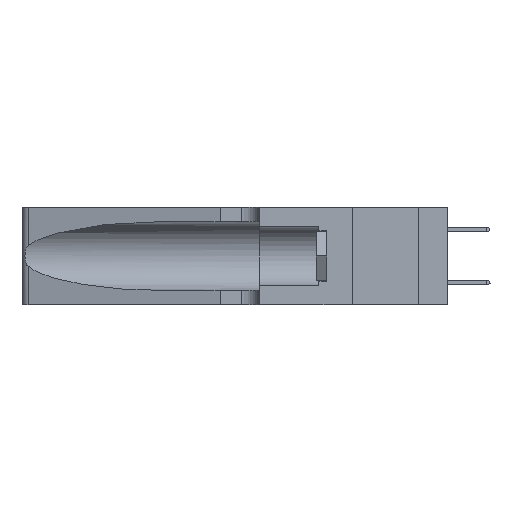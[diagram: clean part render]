
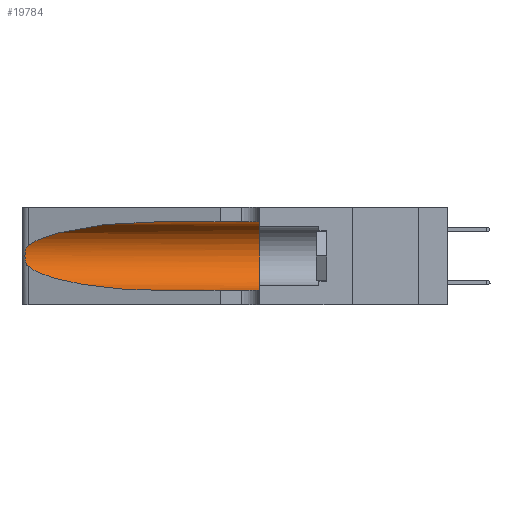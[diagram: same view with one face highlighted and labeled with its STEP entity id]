
A CAD part, left-side view. The second image highlights one B-rep face of the part: STEP entity #19784.
In plain terms, the highlighted cylindrical face has radius 3.308 mm (diameter 6.617 mm), a partial arc.
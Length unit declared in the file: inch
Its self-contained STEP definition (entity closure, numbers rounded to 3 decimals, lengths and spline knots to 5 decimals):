
#1068 = CARTESIAN_POINT ( 'NONE',  ( 0.25856, 1.23593, 0.16098 ) ) ;
#2090 = CARTESIAN_POINT ( 'NONE',  ( 0.1305, 0.35, 0.31525 ) ) ;
#4328 = FACE_OUTER_BOUND ( 'NONE', #12978, .T. ) ;
#4792 = CARTESIAN_POINT ( 'NONE',  ( 0.25487, 1.22718, 0.22369 ) ) ;
#5506 = VERTEX_POINT ( 'NONE', #2090 ) ;
#5895 = EDGE_CURVE ( 'NONE', #29049, #14577, #21340, .T. ) ;
#5913 = CARTESIAN_POINT ( 'NONE',  ( 0.1305, 1.61858, 0.31525 ) ) ;
#6107 = CARTESIAN_POINT ( 'NONE',  ( 0.2373, 1.15595, 0.08982 ) ) ;
#7196 = CARTESIAN_POINT ( 'NONE',  ( 0.25487, 1.22718, 0.22369 ) ) ;
#7689 = CARTESIAN_POINT ( 'NONE',  ( 0.26018, 1.23835, 0.19895 ) ) ;
#8252 = ORIENTED_EDGE ( 'NONE', *, *, #42171, .T. ) ;
#9036 = VECTOR ( 'NONE', #41735, 39.37008 ) ;
#9254 = CARTESIAN_POINT ( 'NONE',  ( 0.2373, 1.15595, 0.28018 ) ) ;
#10290 = CARTESIAN_POINT ( 'NONE',  ( 0.1305, 0.35, 0.185 ) ) ;
#10649 = CARTESIAN_POINT ( 'NONE',  ( 0.25487, 1.22718, 0.22369 ) ) ;
#10930 = CARTESIAN_POINT ( 'NONE',  ( 0.25487, 1.22718, 0.14631 ) ) ;
#11092 = CARTESIAN_POINT ( 'NONE',  ( 0.26075, 1.23896, 0.19203 ) ) ;
#11636 = CARTESIAN_POINT ( 'NONE',  ( 0.1305, 0.72297, 0.05475 ) ) ;
#12978 = EDGE_LOOP ( 'NONE', ( #19654, #16282, #8252, #30655, #33016, #36747 ) ) ;
#13332 = CIRCLE ( 'NONE', #33646, 0.13025 ) ;
#13489 = VERTEX_POINT ( 'NONE', #27936 ) ;
#13955 = CARTESIAN_POINT ( 'NONE',  ( 0.1305, 0.72297, 0.31525 ) ) ;
#13997 = CARTESIAN_POINT ( 'NONE',  ( 0.25639, 1.23186, 0.15144 ) ) ;
#14531 = DIRECTION ( 'NONE',  ( 0., -1., 0. ) ) ;
#14577 = VERTEX_POINT ( 'NONE', #4792 ) ;
#16022 = EDGE_CURVE ( 'NONE', #5506, #13489, #13332, .T. ) ;
#16237 = VECTOR ( 'NONE', #21082, 39.37008 ) ;
#16282 = ORIENTED_EDGE ( 'NONE', *, *, #35152, .T. ) ;
#16532 = DIRECTION ( 'NONE',  ( 0., 1., 0. ) ) ;
#17444 = CARTESIAN_POINT ( 'NONE',  ( 0.25639, 1.23184, 0.21858 ) ) ;
#17752 = CARTESIAN_POINT ( 'NONE',  ( 0.25787, 1.23484, 0.2124 ) ) ;
#18745 = CARTESIAN_POINT ( 'NONE',  ( 0.1305, 0.72297, 0.31525 ) ) ;
#18876 = CARTESIAN_POINT ( 'NONE',  ( 0.25487, 1.22718, 0.14631 ) ) ;
#19654 = ORIENTED_EDGE ( 'NONE', *, *, #5895, .T. ) ;
#19784 = ADVANCED_FACE ( 'NONE', ( #4328 ), #35132, .F. ) ;
#21082 = DIRECTION ( 'NONE',  ( 0., -1., 0. ) ) ;
#21340 =( BOUNDED_CURVE ( )  B_SPLINE_CURVE ( 3, ( #18745, #38522, #9254, #7196 ),
 .UNSPECIFIED., .F., .F. ) 
 B_SPLINE_CURVE_WITH_KNOTS ( ( 4, 4 ),
 ( 1.5708, 2.84003 ),
 .UNSPECIFIED. ) 
 CURVE ( )  GEOMETRIC_REPRESENTATION_ITEM ( )  RATIONAL_B_SPLINE_CURVE ( ( 1., 0.87, 0.87, 1. ) ) 
 REPRESENTATION_ITEM ( '' )  );
#21997 = CARTESIAN_POINT ( 'NONE',  ( 0.1305, 0.72297, 0.05475 ) ) ;
#23235 = DIRECTION ( 'NONE',  ( 0., 0., 1. ) ) ;
#24255 = DIRECTION ( 'NONE',  ( 0., 0., -1. ) ) ;
#24373 = CARTESIAN_POINT ( 'NONE',  ( 0.1305, 1.61858, 0.05475 ) ) ;
#24954 = LINE ( 'NONE', #5913, #9036 ) ;
#25259 = VERTEX_POINT ( 'NONE', #31680 ) ;
#26568 =( BOUNDED_CURVE ( )  B_SPLINE_CURVE ( 3, ( #18876, #6107, #32330, #21997 ),
 .UNSPECIFIED., .F., .F. ) 
 B_SPLINE_CURVE_WITH_KNOTS ( ( 4, 4 ),
 ( 3.44316, 4.71239 ),
 .UNSPECIFIED. ) 
 CURVE ( )  GEOMETRIC_REPRESENTATION_ITEM ( )  RATIONAL_B_SPLINE_CURVE ( ( 1., 0.87, 0.87, 1. ) ) 
 REPRESENTATION_ITEM ( '' )  );
#27039 = CARTESIAN_POINT ( 'NONE',  ( 0.25854, 1.2359, 0.20912 ) ) ;
#27355 = VERTEX_POINT ( 'NONE', #11636 ) ;
#27626 = CARTESIAN_POINT ( 'NONE',  ( 0.25555, 1.22994, 0.2215 ) ) ;
#27936 = CARTESIAN_POINT ( 'NONE',  ( 0.1305, 0.35, 0.05475 ) ) ;
#28009 = CARTESIAN_POINT ( 'NONE',  ( 0.1305, 1.61858, 0.185 ) ) ;
#29049 = VERTEX_POINT ( 'NONE', #13955 ) ;
#30211 = B_SPLINE_CURVE_WITH_KNOTS ( 'NONE', 3,
 ( #10649, #27626, #17444, #17752, #27039, #7689, #11092, #30915, #34252, #1068, #33649, #13997, #30605, #10930 ),
 .UNSPECIFIED., .F., .F.,
 ( 4, 2, 2, 2, 2, 2, 4 ),
 ( 0., 0.00027, 0.00053, 0.00107, 0.0016, 0.00187, 0.00214 ),
 .UNSPECIFIED. ) ;
#30605 = CARTESIAN_POINT ( 'NONE',  ( 0.25555, 1.22993, 0.14849 ) ) ;
#30655 = ORIENTED_EDGE ( 'NONE', *, *, #34658, .T. ) ;
#30915 = CARTESIAN_POINT ( 'NONE',  ( 0.26075, 1.23896, 0.178 ) ) ;
#31680 = CARTESIAN_POINT ( 'NONE',  ( 0.25487, 1.22718, 0.14631 ) ) ;
#32330 = CARTESIAN_POINT ( 'NONE',  ( 0.18966, 0.96281, 0.05475 ) ) ;
#32917 = AXIS2_PLACEMENT_3D ( 'NONE', #28009, #14531, #24255 ) ;
#33016 = ORIENTED_EDGE ( 'NONE', *, *, #16022, .F. ) ;
#33646 = AXIS2_PLACEMENT_3D ( 'NONE', #10290, #16532, #23235 ) ;
#33649 = CARTESIAN_POINT ( 'NONE',  ( 0.25789, 1.23486, 0.15765 ) ) ;
#34252 = CARTESIAN_POINT ( 'NONE',  ( 0.26017, 1.23833, 0.17102 ) ) ;
#34658 = EDGE_CURVE ( 'NONE', #27355, #13489, #35752, .T. ) ;
#34665 = EDGE_CURVE ( 'NONE', #29049, #5506, #24954, .T. ) ;
#35132 = CYLINDRICAL_SURFACE ( 'NONE', #32917, 0.13025 ) ;
#35152 = EDGE_CURVE ( 'NONE', #14577, #25259, #30211, .T. ) ;
#35752 = LINE ( 'NONE', #24373, #16237 ) ;
#36747 = ORIENTED_EDGE ( 'NONE', *, *, #34665, .F. ) ;
#38522 = CARTESIAN_POINT ( 'NONE',  ( 0.18966, 0.96281, 0.31525 ) ) ;
#41735 = DIRECTION ( 'NONE',  ( 0., -1., 0. ) ) ;
#42171 = EDGE_CURVE ( 'NONE', #25259, #27355, #26568, .T. ) ;
